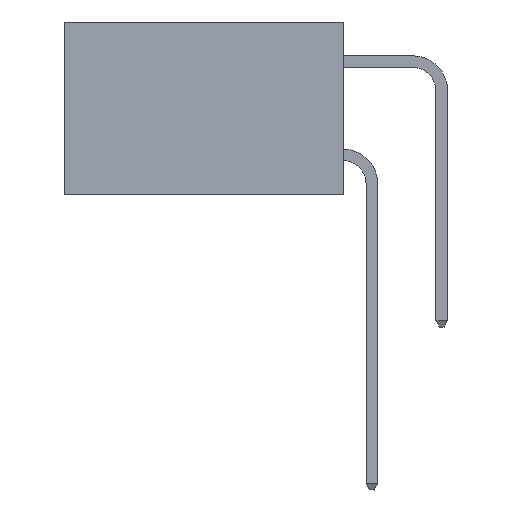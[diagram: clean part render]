
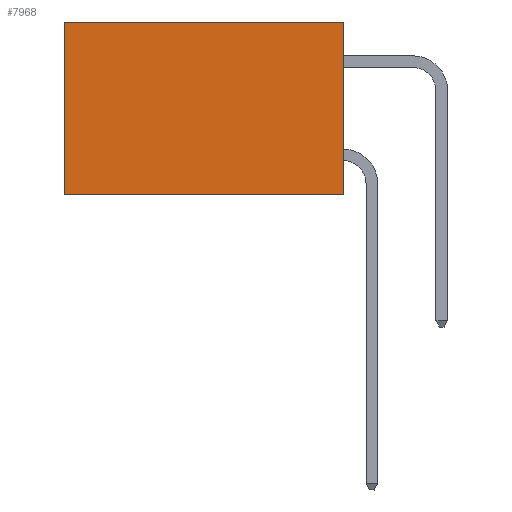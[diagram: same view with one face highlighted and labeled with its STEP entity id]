
A CAD part, left-side view. The second image highlights one B-rep face of the part: STEP entity #7968.
In plain terms, the highlighted planar face has unit normal (-1, 0, 0).
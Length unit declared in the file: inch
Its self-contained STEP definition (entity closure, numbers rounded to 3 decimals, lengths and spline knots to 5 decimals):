
#72 = DIRECTION ( 'NONE',  ( 0., 0., -1. ) ) ;
#472 = EDGE_CURVE ( 'NONE', #15210, #3184, #8602, .T. ) ;
#584 = ORIENTED_EDGE ( 'NONE', *, *, #472, .T. ) ;
#3184 = VERTEX_POINT ( 'NONE', #7240 ) ;
#3270 = VECTOR ( 'NONE', #22045, 39.37008 ) ;
#3686 = CARTESIAN_POINT ( 'NONE',  ( 0.2615, 0., -0.37 ) ) ;
#4122 = EDGE_CURVE ( 'NONE', #20030, #3184, #20540, .T. ) ;
#4190 = CARTESIAN_POINT ( 'NONE',  ( 0.2615, 0., -0.37 ) ) ;
#4708 = EDGE_CURVE ( 'NONE', #24174, #20030, #12936, .T. ) ;
#5107 = VECTOR ( 'NONE', #21631, 39.37008 ) ;
#6048 = CARTESIAN_POINT ( 'NONE',  ( 0.2615, 0., 0. ) ) ;
#6523 = LINE ( 'NONE', #14055, #5107 ) ;
#7240 = CARTESIAN_POINT ( 'NONE',  ( 0.2615, 0.6, -0.37 ) ) ;
#7762 = PLANE ( 'NONE',  #12533 ) ;
#7968 = ADVANCED_FACE ( 'NONE', ( #17040 ), #7762, .F. ) ;
#8602 = LINE ( 'NONE', #20263, #18389 ) ;
#11710 = DIRECTION ( 'NONE',  ( 1., 0., 0. ) ) ;
#12156 = ORIENTED_EDGE ( 'NONE', *, *, #4122, .F. ) ;
#12190 = CARTESIAN_POINT ( 'NONE',  ( 0.2615, 0.6, 0. ) ) ;
#12533 = AXIS2_PLACEMENT_3D ( 'NONE', #4190, #11710, #15306 ) ;
#12870 = EDGE_CURVE ( 'NONE', #24174, #15210, #6523, .T. ) ;
#12936 = LINE ( 'NONE', #3686, #24248 ) ;
#14055 = CARTESIAN_POINT ( 'NONE',  ( 0.2615, 0., 0. ) ) ;
#14817 = EDGE_LOOP ( 'NONE', ( #584, #12156, #17485, #20182 ) ) ;
#14853 = CARTESIAN_POINT ( 'NONE',  ( 0.2615, 0., -0.37 ) ) ;
#15210 = VERTEX_POINT ( 'NONE', #12190 ) ;
#15306 = DIRECTION ( 'NONE',  ( 0., 0., -1. ) ) ;
#16541 = DIRECTION ( 'NONE',  ( 0., 0., -1. ) ) ;
#17040 = FACE_OUTER_BOUND ( 'NONE', #14817, .T. ) ;
#17485 = ORIENTED_EDGE ( 'NONE', *, *, #4708, .F. ) ;
#18389 = VECTOR ( 'NONE', #16541, 39.37008 ) ;
#19149 = CARTESIAN_POINT ( 'NONE',  ( 0.2615, 0., -0.37 ) ) ;
#20030 = VERTEX_POINT ( 'NONE', #19149 ) ;
#20182 = ORIENTED_EDGE ( 'NONE', *, *, #12870, .T. ) ;
#20263 = CARTESIAN_POINT ( 'NONE',  ( 0.2615, 0.6, -0.37 ) ) ;
#20540 = LINE ( 'NONE', #14853, #3270 ) ;
#21631 = DIRECTION ( 'NONE',  ( 0., 1., 0. ) ) ;
#22045 = DIRECTION ( 'NONE',  ( 0., 1., 0. ) ) ;
#24174 = VERTEX_POINT ( 'NONE', #6048 ) ;
#24248 = VECTOR ( 'NONE', #72, 39.37008 ) ;
